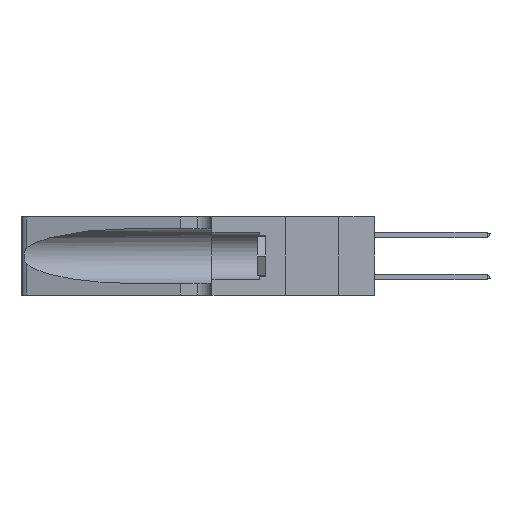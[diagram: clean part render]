
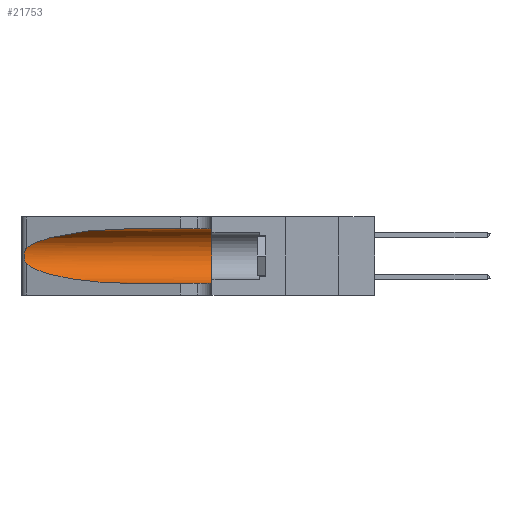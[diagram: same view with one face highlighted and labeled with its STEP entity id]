
A CAD part, left-side view. The second image highlights one B-rep face of the part: STEP entity #21753.
In plain terms, the highlighted cylindrical face has radius 3.308 mm (diameter 6.617 mm), a partial arc.
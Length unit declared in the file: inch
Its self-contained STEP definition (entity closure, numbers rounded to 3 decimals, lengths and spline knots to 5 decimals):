
#267 = CARTESIAN_POINT ( 'NONE',  ( 0.25487, 1.22718, 0.14631 ) ) ;
#581 = CARTESIAN_POINT ( 'NONE',  ( 0.1305, 0.35, 0.185 ) ) ;
#993 = EDGE_CURVE ( 'NONE', #13208, #20422, #1839, .T. ) ;
#1069 = EDGE_LOOP ( 'NONE', ( #6511, #15046, #6826, #11731, #10634, #16584 ) ) ;
#1801 = DIRECTION ( 'NONE',  ( 0., -1., 0. ) ) ;
#1839 = LINE ( 'NONE', #25992, #23334 ) ;
#2161 = DIRECTION ( 'NONE',  ( 0., 0., -1. ) ) ;
#2682 = DIRECTION ( 'NONE',  ( 0., 1., 0. ) ) ;
#3260 = CARTESIAN_POINT ( 'NONE',  ( 0.25555, 1.22994, 0.2215 ) ) ;
#3643 = EDGE_CURVE ( 'NONE', #7499, #17358, #5796, .T. ) ;
#3674 = B_SPLINE_CURVE_WITH_KNOTS ( 'NONE', 3,
 ( #13348, #3260, #11208, #17390, #19435, #23486, #19969, #7859, #22001, #11826, #13956, #9888, #13867, #11378 ),
 .UNSPECIFIED., .F., .F.,
 ( 4, 2, 2, 2, 2, 2, 4 ),
 ( 0., 0.00027, 0.00053, 0.00107, 0.0016, 0.00187, 0.00214 ),
 .UNSPECIFIED. ) ;
#3894 = CARTESIAN_POINT ( 'NONE',  ( 0.2373, 1.15595, 0.08982 ) ) ;
#4126 = CARTESIAN_POINT ( 'NONE',  ( 0.1305, 1.61858, 0.185 ) ) ;
#5066 = CARTESIAN_POINT ( 'NONE',  ( 0.1305, 1.61858, 0.31525 ) ) ;
#5258 = EDGE_CURVE ( 'NONE', #7499, #7758, #24108, .T. ) ;
#5796 = LINE ( 'NONE', #5066, #10875 ) ;
#6122 =( BOUNDED_CURVE ( )  B_SPLINE_CURVE ( 3, ( #20136, #3894, #22086, #15903 ),
 .UNSPECIFIED., .F., .F. ) 
 B_SPLINE_CURVE_WITH_KNOTS ( ( 4, 4 ),
 ( 3.44316, 4.71239 ),
 .UNSPECIFIED. ) 
 CURVE ( )  GEOMETRIC_REPRESENTATION_ITEM ( )  RATIONAL_B_SPLINE_CURVE ( ( 1., 0.87, 0.87, 1. ) ) 
 REPRESENTATION_ITEM ( '' )  );
#6511 = ORIENTED_EDGE ( 'NONE', *, *, #5258, .T. ) ;
#6826 = ORIENTED_EDGE ( 'NONE', *, *, #17580, .T. ) ;
#6955 = CIRCLE ( 'NONE', #21023, 0.13025 ) ;
#7026 = EDGE_CURVE ( 'NONE', #7758, #20508, #3674, .T. ) ;
#7499 = VERTEX_POINT ( 'NONE', #20099 ) ;
#7758 = VERTEX_POINT ( 'NONE', #8241 ) ;
#7859 = CARTESIAN_POINT ( 'NONE',  ( 0.26075, 1.23896, 0.178 ) ) ;
#8241 = CARTESIAN_POINT ( 'NONE',  ( 0.25487, 1.22718, 0.22369 ) ) ;
#8254 = CARTESIAN_POINT ( 'NONE',  ( 0.1305, 0.72297, 0.31525 ) ) ;
#8264 = EDGE_CURVE ( 'NONE', #17358, #20422, #6955, .T. ) ;
#9121 = DIRECTION ( 'NONE',  ( 0., -1., 0. ) ) ;
#9888 = CARTESIAN_POINT ( 'NONE',  ( 0.25639, 1.23186, 0.15144 ) ) ;
#10634 = ORIENTED_EDGE ( 'NONE', *, *, #8264, .F. ) ;
#10875 = VECTOR ( 'NONE', #9121, 39.37008 ) ;
#11208 = CARTESIAN_POINT ( 'NONE',  ( 0.25639, 1.23184, 0.21858 ) ) ;
#11378 = CARTESIAN_POINT ( 'NONE',  ( 0.25487, 1.22718, 0.14631 ) ) ;
#11731 = ORIENTED_EDGE ( 'NONE', *, *, #993, .T. ) ;
#11826 = CARTESIAN_POINT ( 'NONE',  ( 0.25856, 1.23593, 0.16098 ) ) ;
#11924 = DIRECTION ( 'NONE',  ( 0., -1., 0. ) ) ;
#11967 = CARTESIAN_POINT ( 'NONE',  ( 0.25487, 1.22718, 0.22369 ) ) ;
#12790 = AXIS2_PLACEMENT_3D ( 'NONE', #4126, #1801, #2161 ) ;
#13093 = CARTESIAN_POINT ( 'NONE',  ( 0.1305, 0.35, 0.31525 ) ) ;
#13208 = VERTEX_POINT ( 'NONE', #14203 ) ;
#13348 = CARTESIAN_POINT ( 'NONE',  ( 0.25487, 1.22718, 0.22369 ) ) ;
#13867 = CARTESIAN_POINT ( 'NONE',  ( 0.25555, 1.22993, 0.14849 ) ) ;
#13918 = CARTESIAN_POINT ( 'NONE',  ( 0.18966, 0.96281, 0.31525 ) ) ;
#13956 = CARTESIAN_POINT ( 'NONE',  ( 0.25789, 1.23486, 0.15765 ) ) ;
#14203 = CARTESIAN_POINT ( 'NONE',  ( 0.1305, 0.72297, 0.05475 ) ) ;
#15046 = ORIENTED_EDGE ( 'NONE', *, *, #7026, .T. ) ;
#15903 = CARTESIAN_POINT ( 'NONE',  ( 0.1305, 0.72297, 0.05475 ) ) ;
#16584 = ORIENTED_EDGE ( 'NONE', *, *, #3643, .F. ) ;
#17358 = VERTEX_POINT ( 'NONE', #13093 ) ;
#17390 = CARTESIAN_POINT ( 'NONE',  ( 0.25787, 1.23484, 0.2124 ) ) ;
#17580 = EDGE_CURVE ( 'NONE', #20508, #13208, #6122, .T. ) ;
#19435 = CARTESIAN_POINT ( 'NONE',  ( 0.25854, 1.2359, 0.20912 ) ) ;
#19827 = FACE_OUTER_BOUND ( 'NONE', #1069, .T. ) ;
#19969 = CARTESIAN_POINT ( 'NONE',  ( 0.26075, 1.23896, 0.19203 ) ) ;
#20099 = CARTESIAN_POINT ( 'NONE',  ( 0.1305, 0.72297, 0.31525 ) ) ;
#20136 = CARTESIAN_POINT ( 'NONE',  ( 0.25487, 1.22718, 0.14631 ) ) ;
#20422 = VERTEX_POINT ( 'NONE', #24036 ) ;
#20508 = VERTEX_POINT ( 'NONE', #267 ) ;
#20814 = DIRECTION ( 'NONE',  ( 0., 0., 1. ) ) ;
#21023 = AXIS2_PLACEMENT_3D ( 'NONE', #581, #2682, #20814 ) ;
#21753 = ADVANCED_FACE ( 'NONE', ( #19827 ), #25201, .F. ) ;
#22001 = CARTESIAN_POINT ( 'NONE',  ( 0.26017, 1.23833, 0.17102 ) ) ;
#22086 = CARTESIAN_POINT ( 'NONE',  ( 0.18966, 0.96281, 0.05475 ) ) ;
#23334 = VECTOR ( 'NONE', #11924, 39.37008 ) ;
#23486 = CARTESIAN_POINT ( 'NONE',  ( 0.26018, 1.23835, 0.19895 ) ) ;
#24036 = CARTESIAN_POINT ( 'NONE',  ( 0.1305, 0.35, 0.05475 ) ) ;
#24080 = CARTESIAN_POINT ( 'NONE',  ( 0.2373, 1.15595, 0.28018 ) ) ;
#24108 =( BOUNDED_CURVE ( )  B_SPLINE_CURVE ( 3, ( #8254, #13918, #24080, #11967 ),
 .UNSPECIFIED., .F., .F. ) 
 B_SPLINE_CURVE_WITH_KNOTS ( ( 4, 4 ),
 ( 1.5708, 2.84003 ),
 .UNSPECIFIED. ) 
 CURVE ( )  GEOMETRIC_REPRESENTATION_ITEM ( )  RATIONAL_B_SPLINE_CURVE ( ( 1., 0.87, 0.87, 1. ) ) 
 REPRESENTATION_ITEM ( '' )  );
#25201 = CYLINDRICAL_SURFACE ( 'NONE', #12790, 0.13025 ) ;
#25992 = CARTESIAN_POINT ( 'NONE',  ( 0.1305, 1.61858, 0.05475 ) ) ;
